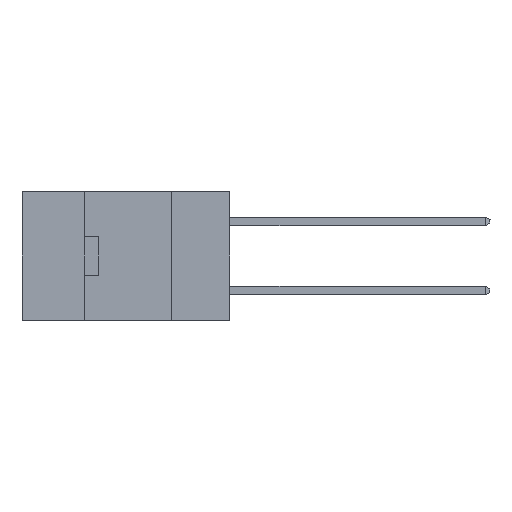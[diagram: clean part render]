
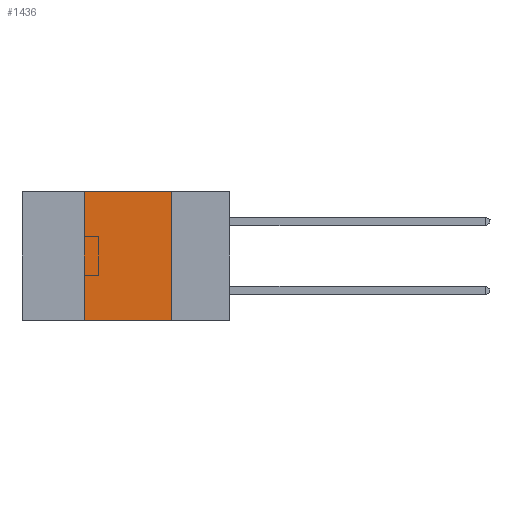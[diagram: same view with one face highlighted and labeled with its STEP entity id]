
A CAD part, left-side view. The second image highlights one B-rep face of the part: STEP entity #1436.
In plain terms, the highlighted planar face has unit normal (-1, 0, 0).
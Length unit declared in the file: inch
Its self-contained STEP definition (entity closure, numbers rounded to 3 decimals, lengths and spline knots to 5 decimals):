
#233 = LINE ( 'NONE', #20137, #10466 ) ;
#367 = VERTEX_POINT ( 'NONE', #17117 ) ;
#973 = DIRECTION ( 'NONE',  ( 0., -1., 0. ) ) ;
#1436 = ADVANCED_FACE ( 'NONE', ( #16715 ), #28063, .F. ) ;
#4597 = DIRECTION ( 'NONE',  ( 0., -1., 0. ) ) ;
#5937 = LINE ( 'NONE', #13992, #9820 ) ;
#6954 = ORIENTED_EDGE ( 'NONE', *, *, #10120, .F. ) ;
#7671 = CARTESIAN_POINT ( 'NONE',  ( 0., 0.6, -0.37 ) ) ;
#7900 = ORIENTED_EDGE ( 'NONE', *, *, #9166, .F. ) ;
#8157 = CARTESIAN_POINT ( 'NONE',  ( 0., 0.6, 0. ) ) ;
#9166 = EDGE_CURVE ( 'NONE', #367, #11678, #5937, .T. ) ;
#9820 = VECTOR ( 'NONE', #14802, 39.37008 ) ;
#10120 = EDGE_CURVE ( 'NONE', #10155, #19823, #18651, .T. ) ;
#10155 = VERTEX_POINT ( 'NONE', #15780 ) ;
#10466 = VECTOR ( 'NONE', #4597, 39.37008 ) ;
#11242 = EDGE_LOOP ( 'NONE', ( #7900, #17739, #6954, #22612 ) ) ;
#11317 = CARTESIAN_POINT ( 'NONE',  ( 0., 0.42, 0. ) ) ;
#11678 = VERTEX_POINT ( 'NONE', #27990 ) ;
#12328 = LINE ( 'NONE', #7671, #16905 ) ;
#13618 = CARTESIAN_POINT ( 'NONE',  ( 0., 0.42, -0.37 ) ) ;
#13992 = CARTESIAN_POINT ( 'NONE',  ( 0., 0.17, -0.37 ) ) ;
#14802 = DIRECTION ( 'NONE',  ( 0., 0., -1. ) ) ;
#14826 = DIRECTION ( 'NONE',  ( 1., 0., 0. ) ) ;
#15780 = CARTESIAN_POINT ( 'NONE',  ( 0., 0.42, -0.37 ) ) ;
#16715 = FACE_OUTER_BOUND ( 'NONE', #11242, .T. ) ;
#16905 = VECTOR ( 'NONE', #973, 39.37008 ) ;
#17017 = DIRECTION ( 'NONE',  ( 0., 0., -1. ) ) ;
#17117 = CARTESIAN_POINT ( 'NONE',  ( 0., 0.17, 0. ) ) ;
#17739 = ORIENTED_EDGE ( 'NONE', *, *, #21565, .F. ) ;
#18651 = LINE ( 'NONE', #13618, #23545 ) ;
#19823 = VERTEX_POINT ( 'NONE', #11317 ) ;
#19956 = EDGE_CURVE ( 'NONE', #10155, #11678, #12328, .T. ) ;
#20137 = CARTESIAN_POINT ( 'NONE',  ( 0., 0.6, 0. ) ) ;
#20991 = AXIS2_PLACEMENT_3D ( 'NONE', #8157, #14826, #17017 ) ;
#21565 = EDGE_CURVE ( 'NONE', #19823, #367, #233, .T. ) ;
#22612 = ORIENTED_EDGE ( 'NONE', *, *, #19956, .T. ) ;
#23137 = DIRECTION ( 'NONE',  ( 0., 0., 1. ) ) ;
#23545 = VECTOR ( 'NONE', #23137, 39.37008 ) ;
#27990 = CARTESIAN_POINT ( 'NONE',  ( 0., 0.17, -0.37 ) ) ;
#28063 = PLANE ( 'NONE',  #20991 ) ;
